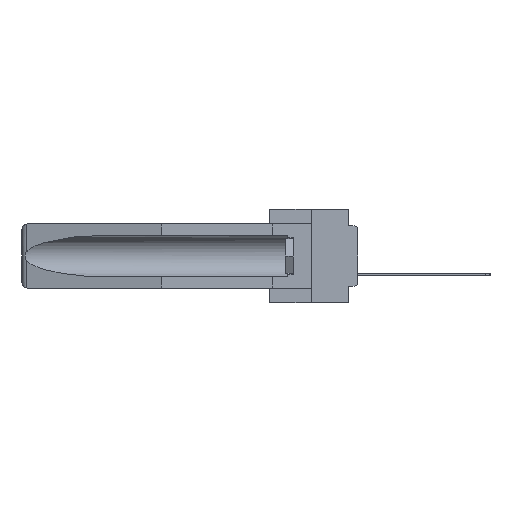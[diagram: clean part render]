
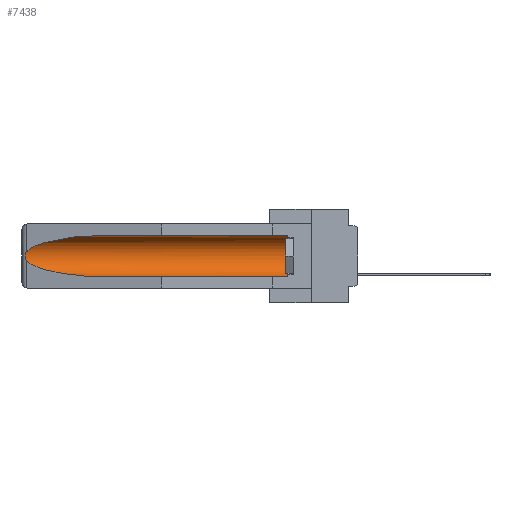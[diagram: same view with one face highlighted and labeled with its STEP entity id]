
A CAD part, left-side view. The second image highlights one B-rep face of the part: STEP entity #7438.
In plain terms, the highlighted cylindrical face has radius 2.857 mm (diameter 5.715 mm), a partial arc.
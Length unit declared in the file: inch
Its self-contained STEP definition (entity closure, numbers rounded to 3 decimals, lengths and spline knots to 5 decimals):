
#1072 = LINE ( 'NONE', #29011, #2322 ) ;
#1274 = CARTESIAN_POINT ( 'NONE',  ( 0.21114, 1.30732, -0.284 ) ) ;
#2134 = ORIENTED_EDGE ( 'NONE', *, *, #3435, .T. ) ;
#2322 = VECTOR ( 'NONE', #29474, 39.37008 ) ;
#3435 = EDGE_CURVE ( 'NONE', #10208, #15731, #5422, .T. ) ;
#3727 = EDGE_CURVE ( 'NONE', #19565, #10986, #9548, .T. ) ;
#4625 = CARTESIAN_POINT ( 'NONE',  ( 0.155, 1.07973, -0.059 ) ) ;
#5003 = AXIS2_PLACEMENT_3D ( 'NONE', #8034, #17432, #12830 ) ;
#5422 =( BOUNDED_CURVE ( )  B_SPLINE_CURVE ( 3, ( #17120, #21845, #1274, #20178 ),
 .UNSPECIFIED., .F., .F. ) 
 B_SPLINE_CURVE_WITH_KNOTS ( ( 4, 4 ),
 ( 0.1948, 1.5708 ),
 .UNSPECIFIED. ) 
 CURVE ( )  GEOMETRIC_REPRESENTATION_ITEM ( )  RATIONAL_B_SPLINE_CURVE ( ( 1., 0.848, 0.848, 1. ) ) 
 REPRESENTATION_ITEM ( '' )  );
#5839 = CARTESIAN_POINT ( 'NONE',  ( 0.26537, 1.52718, -0.14972 ) ) ;
#6974 = CARTESIAN_POINT ( 'NONE',  ( 0.26537, 1.52718, -0.19328 ) ) ;
#7438 = ADVANCED_FACE ( 'NONE', ( #24294 ), #12680, .F. ) ;
#8034 = CARTESIAN_POINT ( 'NONE',  ( 0.155, -0.30754, -0.1715 ) ) ;
#9434 = CARTESIAN_POINT ( 'NONE',  ( 0.26655, 1.53094, -0.18657 ) ) ;
#9548 =( BOUNDED_CURVE ( )  B_SPLINE_CURVE ( 3, ( #4625, #26556, #26860, #5839 ),
 .UNSPECIFIED., .F., .F. ) 
 B_SPLINE_CURVE_WITH_KNOTS ( ( 4, 4 ),
 ( 4.71239, 6.08839 ),
 .UNSPECIFIED. ) 
 CURVE ( )  GEOMETRIC_REPRESENTATION_ITEM ( )  RATIONAL_B_SPLINE_CURVE ( ( 1., 0.848, 0.848, 1. ) ) 
 REPRESENTATION_ITEM ( '' )  );
#9855 = CARTESIAN_POINT ( 'NONE',  ( 0.155, 0.126, -0.059 ) ) ;
#10208 = VERTEX_POINT ( 'NONE', #23106 ) ;
#10622 = EDGE_LOOP ( 'NONE', ( #25273, #29824, #2134, #20764, #15687, #24590 ) ) ;
#10986 = VERTEX_POINT ( 'NONE', #28892 ) ;
#11409 = CIRCLE ( 'NONE', #28559, 0.1125 ) ;
#11596 = CARTESIAN_POINT ( 'NONE',  ( 0.26537, 1.52718, -0.14972 ) ) ;
#11914 = CARTESIAN_POINT ( 'NONE',  ( 0.26654, 1.53092, -0.15636 ) ) ;
#12047 = EDGE_CURVE ( 'NONE', #10986, #10208, #20519, .T. ) ;
#12680 = CYLINDRICAL_SURFACE ( 'NONE', #5003, 0.1125 ) ;
#12830 = DIRECTION ( 'NONE',  ( 0., 0., 1. ) ) ;
#15137 = DIRECTION ( 'NONE',  ( 0., 1., 0. ) ) ;
#15687 = ORIENTED_EDGE ( 'NONE', *, *, #20721, .T. ) ;
#15731 = VERTEX_POINT ( 'NONE', #21711 ) ;
#16140 = EDGE_CURVE ( 'NONE', #27316, #19565, #1072, .T. ) ;
#16512 = CARTESIAN_POINT ( 'NONE',  ( 0.2675, 1.53308, -0.17534 ) ) ;
#17069 = EDGE_CURVE ( 'NONE', #19715, #15731, #26759, .T. ) ;
#17120 = CARTESIAN_POINT ( 'NONE',  ( 0.26537, 1.52718, -0.19328 ) ) ;
#17432 = DIRECTION ( 'NONE',  ( 0., 1., 0. ) ) ;
#17486 = CARTESIAN_POINT ( 'NONE',  ( 0.155, 0.126, -0.1715 ) ) ;
#18970 = CARTESIAN_POINT ( 'NONE',  ( 0.2675, 1.53308, -0.16763 ) ) ;
#19069 = VECTOR ( 'NONE', #15137, 39.37008 ) ;
#19565 = VERTEX_POINT ( 'NONE', #24801 ) ;
#19715 = VERTEX_POINT ( 'NONE', #25548 ) ;
#20178 = CARTESIAN_POINT ( 'NONE',  ( 0.155, 1.07973, -0.284 ) ) ;
#20519 = B_SPLINE_CURVE_WITH_KNOTS ( 'NONE', 3,
 ( #11596, #23398, #11914, #30315, #18970, #16512, #28308, #9434, #25697, #6974 ),
 .UNSPECIFIED., .F., .F.,
 ( 4, 2, 2, 2, 4 ),
 ( 0., 0.00029, 0.00058, 0.00087, 0.00117 ),
 .UNSPECIFIED. ) ;
#20721 = EDGE_CURVE ( 'NONE', #19715, #27316, #11409, .T. ) ;
#20764 = ORIENTED_EDGE ( 'NONE', *, *, #17069, .F. ) ;
#21711 = CARTESIAN_POINT ( 'NONE',  ( 0.155, 1.07973, -0.284 ) ) ;
#21845 = CARTESIAN_POINT ( 'NONE',  ( 0.25451, 1.48313, -0.24835 ) ) ;
#21901 = DIRECTION ( 'NONE',  ( 0., 0., 1. ) ) ;
#23106 = CARTESIAN_POINT ( 'NONE',  ( 0.26537, 1.52718, -0.19328 ) ) ;
#23398 = CARTESIAN_POINT ( 'NONE',  ( 0.26597, 1.52961, -0.15275 ) ) ;
#24294 = FACE_OUTER_BOUND ( 'NONE', #10622, .T. ) ;
#24590 = ORIENTED_EDGE ( 'NONE', *, *, #16140, .T. ) ;
#24801 = CARTESIAN_POINT ( 'NONE',  ( 0.155, 1.07973, -0.059 ) ) ;
#25273 = ORIENTED_EDGE ( 'NONE', *, *, #3727, .T. ) ;
#25548 = CARTESIAN_POINT ( 'NONE',  ( 0.155, 0.126, -0.284 ) ) ;
#25697 = CARTESIAN_POINT ( 'NONE',  ( 0.26597, 1.5296, -0.19026 ) ) ;
#26556 = CARTESIAN_POINT ( 'NONE',  ( 0.21114, 1.30732, -0.059 ) ) ;
#26759 = LINE ( 'NONE', #28633, #19069 ) ;
#26860 = CARTESIAN_POINT ( 'NONE',  ( 0.25451, 1.48313, -0.09465 ) ) ;
#27316 = VERTEX_POINT ( 'NONE', #9855 ) ;
#28308 = CARTESIAN_POINT ( 'NONE',  ( 0.2673, 1.53269, -0.17917 ) ) ;
#28514 = DIRECTION ( 'NONE',  ( 0., -1., 0. ) ) ;
#28559 = AXIS2_PLACEMENT_3D ( 'NONE', #17486, #28514, #21901 ) ;
#28633 = CARTESIAN_POINT ( 'NONE',  ( 0.155, -0.30754, -0.284 ) ) ;
#28892 = CARTESIAN_POINT ( 'NONE',  ( 0.26537, 1.52718, -0.14972 ) ) ;
#29011 = CARTESIAN_POINT ( 'NONE',  ( 0.155, -0.30754, -0.059 ) ) ;
#29474 = DIRECTION ( 'NONE',  ( 0., 1., 0. ) ) ;
#29824 = ORIENTED_EDGE ( 'NONE', *, *, #12047, .T. ) ;
#30315 = CARTESIAN_POINT ( 'NONE',  ( 0.2673, 1.5327, -0.16383 ) ) ;
